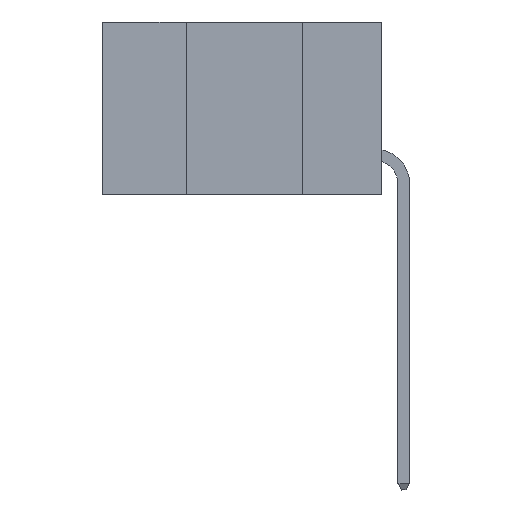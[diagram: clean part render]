
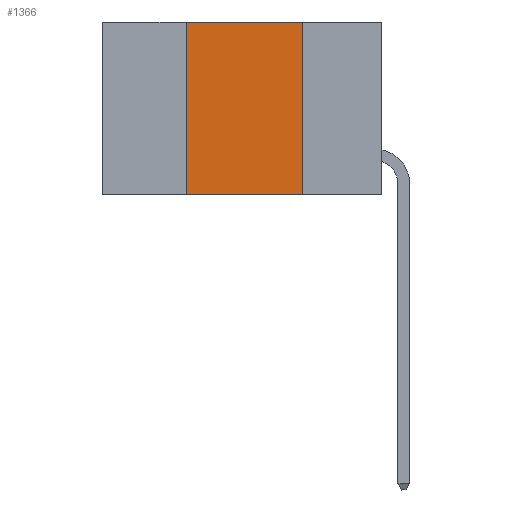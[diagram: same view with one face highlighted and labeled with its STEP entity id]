
A CAD part, left-side view. The second image highlights one B-rep face of the part: STEP entity #1366.
In plain terms, the highlighted planar face has unit normal (-1, 0, 0).
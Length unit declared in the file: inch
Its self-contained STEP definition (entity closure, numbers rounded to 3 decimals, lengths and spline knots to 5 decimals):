
#1366 = ADVANCED_FACE ( 'NONE', ( #7666 ), #30619, .F. ) ;
#5139 = DIRECTION ( 'NONE',  ( 0., -1., 0. ) ) ;
#5514 = CARTESIAN_POINT ( 'NONE',  ( 0., 0.42, 0. ) ) ;
#5951 = VECTOR ( 'NONE', #8757, 39.37008 ) ;
#7666 = FACE_OUTER_BOUND ( 'NONE', #32353, .T. ) ;
#8113 = VERTEX_POINT ( 'NONE', #38664 ) ;
#8757 = DIRECTION ( 'NONE',  ( 0., 0., -1. ) ) ;
#9562 = CARTESIAN_POINT ( 'NONE',  ( 0., 0.17, 0. ) ) ;
#10273 = DIRECTION ( 'NONE',  ( 1., 0., 0. ) ) ;
#12325 = LINE ( 'NONE', #31268, #5951 ) ;
#15305 = ORIENTED_EDGE ( 'NONE', *, *, #36852, .F. ) ;
#19906 = AXIS2_PLACEMENT_3D ( 'NONE', #30482, #10273, #30756 ) ;
#19994 = EDGE_CURVE ( 'NONE', #32346, #21143, #35600, .T. ) ;
#20230 = LINE ( 'NONE', #29644, #36275 ) ;
#20469 = VECTOR ( 'NONE', #5139, 39.37008 ) ;
#21143 = VERTEX_POINT ( 'NONE', #5514 ) ;
#22758 = DIRECTION ( 'NONE',  ( 0., -1., 0. ) ) ;
#24372 = DIRECTION ( 'NONE',  ( 0., 0., 1. ) ) ;
#26016 = VERTEX_POINT ( 'NONE', #9562 ) ;
#26540 = VECTOR ( 'NONE', #24372, 39.37008 ) ;
#27049 = ORIENTED_EDGE ( 'NONE', *, *, #19994, .F. ) ;
#29018 = ORIENTED_EDGE ( 'NONE', *, *, #29808, .F. ) ;
#29644 = CARTESIAN_POINT ( 'NONE',  ( 0., 0.6, 0. ) ) ;
#29808 = EDGE_CURVE ( 'NONE', #21143, #26016, #20230, .T. ) ;
#30482 = CARTESIAN_POINT ( 'NONE',  ( 0., 0.6, 0. ) ) ;
#30619 = PLANE ( 'NONE',  #19906 ) ;
#30756 = DIRECTION ( 'NONE',  ( 0., 0., -1. ) ) ;
#31268 = CARTESIAN_POINT ( 'NONE',  ( 0., 0.17, 0. ) ) ;
#32346 = VERTEX_POINT ( 'NONE', #38680 ) ;
#32353 = EDGE_LOOP ( 'NONE', ( #15305, #29018, #27049, #37481 ) ) ;
#33301 = LINE ( 'NONE', #35161, #20469 ) ;
#33527 = EDGE_CURVE ( 'NONE', #32346, #8113, #33301, .T. ) ;
#34977 = CARTESIAN_POINT ( 'NONE',  ( 0., 0.42, 0. ) ) ;
#35161 = CARTESIAN_POINT ( 'NONE',  ( 0., 0.6, -0.37 ) ) ;
#35600 = LINE ( 'NONE', #34977, #26540 ) ;
#36275 = VECTOR ( 'NONE', #22758, 39.37008 ) ;
#36852 = EDGE_CURVE ( 'NONE', #26016, #8113, #12325, .T. ) ;
#37481 = ORIENTED_EDGE ( 'NONE', *, *, #33527, .T. ) ;
#38664 = CARTESIAN_POINT ( 'NONE',  ( 0., 0.17, -0.37 ) ) ;
#38680 = CARTESIAN_POINT ( 'NONE',  ( 0., 0.42, -0.37 ) ) ;
